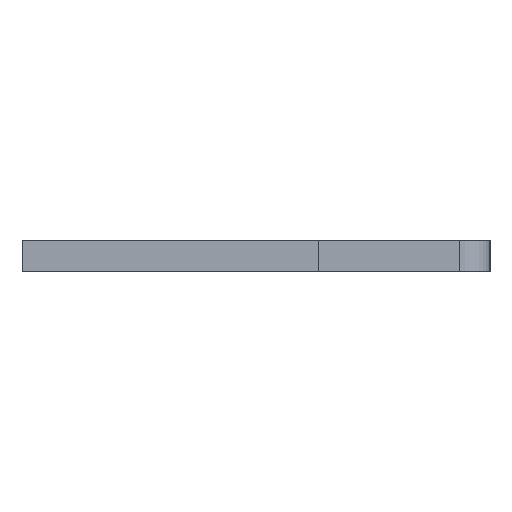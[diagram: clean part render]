
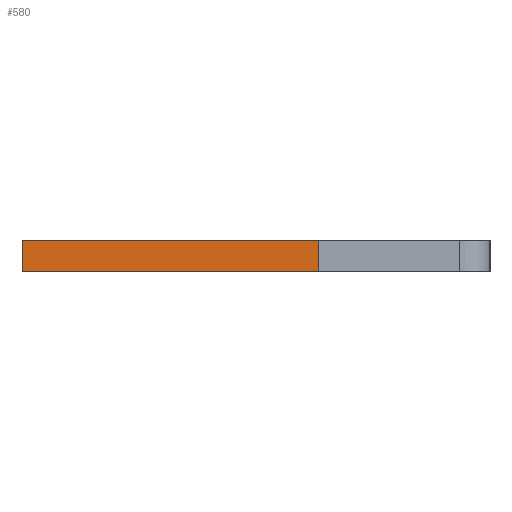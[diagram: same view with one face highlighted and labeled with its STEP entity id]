
A CAD part, left-side view. The second image highlights one B-rep face of the part: STEP entity #580.
In plain terms, the highlighted face is planar.
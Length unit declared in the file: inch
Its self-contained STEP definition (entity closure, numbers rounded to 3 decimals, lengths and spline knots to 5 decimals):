
#7 = VECTOR ( 'NONE', #1023, 39.37008 ) ;
#31 = ORIENTED_EDGE ( 'NONE', *, *, #874, .F. ) ;
#35 = CARTESIAN_POINT ( 'NONE',  ( -0.01, -0.04, -0.04 ) ) ;
#79 = CARTESIAN_POINT ( 'NONE',  ( -0.01, 0.15, -0.04 ) ) ;
#85 = CARTESIAN_POINT ( 'NONE',  ( 0.01, 0.15, -0.04 ) ) ;
#255 = AXIS2_PLACEMENT_3D ( 'NONE', #85, #1429, #1585 ) ;
#300 = EDGE_CURVE ( 'NONE', #547, #528, #725, .T. ) ;
#307 = FACE_OUTER_BOUND ( 'NONE', #1259, .T. ) ;
#482 = CARTESIAN_POINT ( 'NONE',  ( 0.01, -0.04, -0.04 ) ) ;
#528 = VERTEX_POINT ( 'NONE', #79 ) ;
#547 = VERTEX_POINT ( 'NONE', #1563 ) ;
#580 = ADVANCED_FACE ( 'NONE', ( #307 ), #840, .F. ) ;
#610 = LINE ( 'NONE', #1010, #913 ) ;
#669 = EDGE_CURVE ( 'NONE', #1751, #528, #1195, .T. ) ;
#725 = LINE ( 'NONE', #1830, #1006 ) ;
#840 = PLANE ( 'NONE',  #255 ) ;
#874 = EDGE_CURVE ( 'NONE', #1583, #547, #610, .T. ) ;
#899 = DIRECTION ( 'NONE',  ( 0., 1., 0. ) ) ;
#913 = VECTOR ( 'NONE', #899, 39.37008 ) ;
#923 = CARTESIAN_POINT ( 'NONE',  ( 0.01, -0.04, -0.04 ) ) ;
#1006 = VECTOR ( 'NONE', #1390, 39.37008 ) ;
#1010 = CARTESIAN_POINT ( 'NONE',  ( 0.01, 0.15, -0.04 ) ) ;
#1023 = DIRECTION ( 'NONE',  ( 0., 1., 0. ) ) ;
#1026 = VECTOR ( 'NONE', #1222, 39.37008 ) ;
#1195 = LINE ( 'NONE', #1453, #7 ) ;
#1206 = ORIENTED_EDGE ( 'NONE', *, *, #300, .F. ) ;
#1222 = DIRECTION ( 'NONE',  ( -1., 0., 0. ) ) ;
#1259 = EDGE_LOOP ( 'NONE', ( #1868, #1206, #31, #1656 ) ) ;
#1390 = DIRECTION ( 'NONE',  ( -1., 0., 0. ) ) ;
#1429 = DIRECTION ( 'NONE',  ( 0., 0., 1. ) ) ;
#1453 = CARTESIAN_POINT ( 'NONE',  ( -0.01, 0.15, -0.04 ) ) ;
#1501 = LINE ( 'NONE', #923, #1026 ) ;
#1563 = CARTESIAN_POINT ( 'NONE',  ( 0.01, 0.15, -0.04 ) ) ;
#1583 = VERTEX_POINT ( 'NONE', #482 ) ;
#1585 = DIRECTION ( 'NONE',  ( 1., 0., 0. ) ) ;
#1656 = ORIENTED_EDGE ( 'NONE', *, *, #1666, .T. ) ;
#1666 = EDGE_CURVE ( 'NONE', #1583, #1751, #1501, .T. ) ;
#1751 = VERTEX_POINT ( 'NONE', #35 ) ;
#1830 = CARTESIAN_POINT ( 'NONE',  ( 0.01, 0.15, -0.04 ) ) ;
#1868 = ORIENTED_EDGE ( 'NONE', *, *, #669, .T. ) ;
